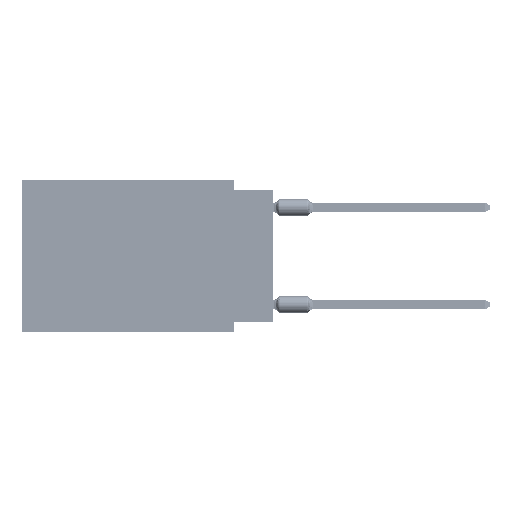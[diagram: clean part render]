
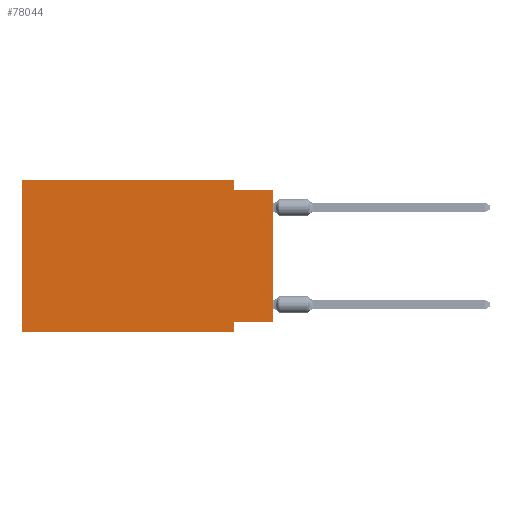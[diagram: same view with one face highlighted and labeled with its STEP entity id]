
A CAD part, left-side view. The second image highlights one B-rep face of the part: STEP entity #78044.
In plain terms, the highlighted planar face has unit normal (-1, 0, 0).
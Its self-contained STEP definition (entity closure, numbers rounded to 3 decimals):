
#901 = AXIS2_PLACEMENT_3D ( 'NONE', #18094, #84283, #43726 ) ;
#2890 = CARTESIAN_POINT ( 'NONE',  ( 0., 16.383, 0. ) ) ;
#4146 = DIRECTION ( 'NONE',  ( 0., 0., 1. ) ) ;
#6298 = EDGE_CURVE ( 'NONE', #51844, #35221, #28367, .T. ) ;
#8703 = CARTESIAN_POINT ( 'NONE',  ( 0., 0., -0.635 ) ) ;
#9265 = DIRECTION ( 'NONE',  ( 0., 1., 0. ) ) ;
#9777 = VERTEX_POINT ( 'NONE', #8703 ) ;
#10093 = LINE ( 'NONE', #75028, #66871 ) ;
#16290 = VECTOR ( 'NONE', #4146, 1000. ) ;
#17525 = EDGE_CURVE ( 'NONE', #65732, #66290, #46840, .T. ) ;
#18094 = CARTESIAN_POINT ( 'NONE',  ( 0., 16.383, 0. ) ) ;
#19801 = EDGE_CURVE ( 'NONE', #50804, #9777, #71064, .T. ) ;
#22421 = CARTESIAN_POINT ( 'NONE',  ( 0., 2.54, 0. ) ) ;
#24320 = ORIENTED_EDGE ( 'NONE', *, *, #56542, .T. ) ;
#25870 = VECTOR ( 'NONE', #83022, 1000. ) ;
#27775 = ORIENTED_EDGE ( 'NONE', *, *, #56322, .F. ) ;
#28084 = CARTESIAN_POINT ( 'NONE',  ( 0., 2.54, -9.906 ) ) ;
#28367 = LINE ( 'NONE', #41618, #30632 ) ;
#29205 = VERTEX_POINT ( 'NONE', #80720 ) ;
#30632 = VECTOR ( 'NONE', #48026, 1000. ) ;
#31166 = DIRECTION ( 'NONE',  ( 0., 0., -1. ) ) ;
#34152 = ORIENTED_EDGE ( 'NONE', *, *, #17525, .F. ) ;
#34829 = VECTOR ( 'NONE', #9265, 1000. ) ;
#35221 = VERTEX_POINT ( 'NONE', #22421 ) ;
#35332 = LINE ( 'NONE', #82286, #34829 ) ;
#35832 = DIRECTION ( 'NONE',  ( 0., -1., 0. ) ) ;
#36618 = LINE ( 'NONE', #2890, #16290 ) ;
#36996 = VECTOR ( 'NONE', #35832, 1000. ) ;
#41384 = LINE ( 'NONE', #67450, #36996 ) ;
#41618 = CARTESIAN_POINT ( 'NONE',  ( 0., 16.383, 0. ) ) ;
#43726 = DIRECTION ( 'NONE',  ( 0., 0., -1. ) ) ;
#44147 = CARTESIAN_POINT ( 'NONE',  ( 0., 0., -0.635 ) ) ;
#46840 = LINE ( 'NONE', #72922, #58569 ) ;
#48026 = DIRECTION ( 'NONE',  ( 0., -1., 0. ) ) ;
#50804 = VERTEX_POINT ( 'NONE', #61639 ) ;
#51844 = VERTEX_POINT ( 'NONE', #68343 ) ;
#51987 = VECTOR ( 'NONE', #71339, 1000. ) ;
#54303 = ORIENTED_EDGE ( 'NONE', *, *, #76287, .F. ) ;
#54782 = EDGE_CURVE ( 'NONE', #76879, #9777, #10093, .T. ) ;
#56322 = EDGE_CURVE ( 'NONE', #35221, #50804, #83709, .T. ) ;
#56542 = EDGE_CURVE ( 'NONE', #29205, #66290, #41384, .T. ) ;
#58565 = CARTESIAN_POINT ( 'NONE',  ( 0., 2.54, -9.271 ) ) ;
#58569 = VECTOR ( 'NONE', #31166, 1000. ) ;
#59183 = ORIENTED_EDGE ( 'NONE', *, *, #6298, .F. ) ;
#60794 = ORIENTED_EDGE ( 'NONE', *, *, #68106, .F. ) ;
#61639 = CARTESIAN_POINT ( 'NONE',  ( 0., 2.54, -0.635 ) ) ;
#63604 = EDGE_LOOP ( 'NONE', ( #68724, #82540, #27775, #59183, #60794, #24320, #34152, #54303 ) ) ;
#64232 = FACE_OUTER_BOUND ( 'NONE', #63604, .T. ) ;
#65732 = VERTEX_POINT ( 'NONE', #58565 ) ;
#66290 = VERTEX_POINT ( 'NONE', #28084 ) ;
#66871 = VECTOR ( 'NONE', #81009, 1000. ) ;
#67450 = CARTESIAN_POINT ( 'NONE',  ( 0., 16.383, -9.906 ) ) ;
#68106 = EDGE_CURVE ( 'NONE', #29205, #51844, #36618, .T. ) ;
#68343 = CARTESIAN_POINT ( 'NONE',  ( 0., 16.383, 0. ) ) ;
#68724 = ORIENTED_EDGE ( 'NONE', *, *, #54782, .T. ) ;
#70626 = CARTESIAN_POINT ( 'NONE',  ( 0., 0., -9.271 ) ) ;
#70636 = PLANE ( 'NONE',  #901 ) ;
#71064 = LINE ( 'NONE', #44147, #25870 ) ;
#71339 = DIRECTION ( 'NONE',  ( 0., 0., -1. ) ) ;
#72922 = CARTESIAN_POINT ( 'NONE',  ( 0., 2.54, -9.906 ) ) ;
#75028 = CARTESIAN_POINT ( 'NONE',  ( 0., 0., 0. ) ) ;
#76287 = EDGE_CURVE ( 'NONE', #76879, #65732, #35332, .T. ) ;
#76879 = VERTEX_POINT ( 'NONE', #70626 ) ;
#77717 = CARTESIAN_POINT ( 'NONE',  ( 0., 2.54, 0. ) ) ;
#78044 = ADVANCED_FACE ( 'NONE', ( #64232 ), #70636, .F. ) ;
#80720 = CARTESIAN_POINT ( 'NONE',  ( 0., 16.383, -9.906 ) ) ;
#81009 = DIRECTION ( 'NONE',  ( 0., 0., 1. ) ) ;
#82286 = CARTESIAN_POINT ( 'NONE',  ( 0., 0., -9.271 ) ) ;
#82540 = ORIENTED_EDGE ( 'NONE', *, *, #19801, .F. ) ;
#83022 = DIRECTION ( 'NONE',  ( 0., -1., 0. ) ) ;
#83709 = LINE ( 'NONE', #77717, #51987 ) ;
#84283 = DIRECTION ( 'NONE',  ( 1., 0., 0. ) ) ;
